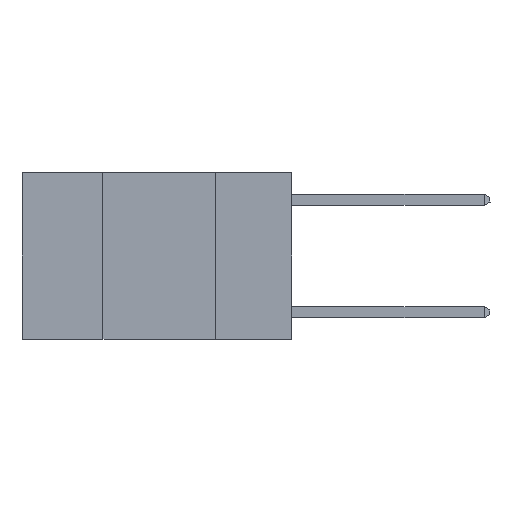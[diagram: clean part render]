
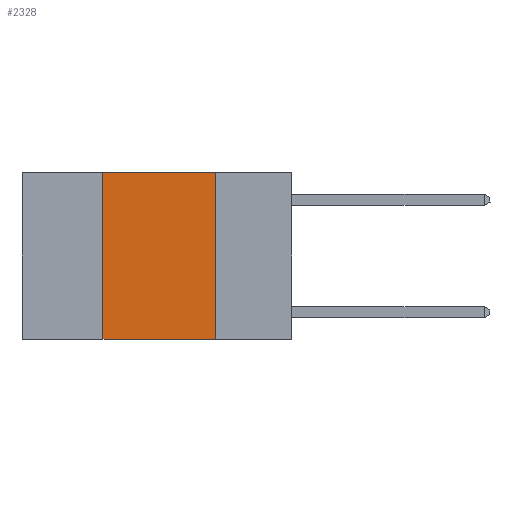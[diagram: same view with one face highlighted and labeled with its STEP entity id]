
A CAD part, left-side view. The second image highlights one B-rep face of the part: STEP entity #2328.
In plain terms, the highlighted planar face has unit normal (-1, 0, 0).
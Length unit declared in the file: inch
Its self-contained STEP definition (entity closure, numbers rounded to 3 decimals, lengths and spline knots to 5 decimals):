
#122 = ORIENTED_EDGE ( 'NONE', *, *, #6256, .F. ) ;
#449 = CARTESIAN_POINT ( 'NONE',  ( 0., 0.42, -0.37 ) ) ;
#525 = LINE ( 'NONE', #4848, #6279 ) ;
#731 = VECTOR ( 'NONE', #2722, 39.37008 ) ;
#1055 = DIRECTION ( 'NONE',  ( 0., -1., 0. ) ) ;
#1073 = CARTESIAN_POINT ( 'NONE',  ( 0., 0.6, -0.37 ) ) ;
#1463 = DIRECTION ( 'NONE',  ( 0., 0., -1. ) ) ;
#1555 = VERTEX_POINT ( 'NONE', #2569 ) ;
#1876 = CARTESIAN_POINT ( 'NONE',  ( 0., 0.42, 0. ) ) ;
#1993 = CARTESIAN_POINT ( 'NONE',  ( 0., 0.6, 0. ) ) ;
#2189 = VERTEX_POINT ( 'NONE', #449 ) ;
#2293 = ORIENTED_EDGE ( 'NONE', *, *, #6608, .F. ) ;
#2328 = ADVANCED_FACE ( 'NONE', ( #3633 ), #8677, .F. ) ;
#2569 = CARTESIAN_POINT ( 'NONE',  ( 0., 0.42, 0. ) ) ;
#2722 = DIRECTION ( 'NONE',  ( 0., 0., 1. ) ) ;
#3633 = FACE_OUTER_BOUND ( 'NONE', #6248, .T. ) ;
#3736 = EDGE_CURVE ( 'NONE', #2189, #7300, #4360, .T. ) ;
#3744 = CARTESIAN_POINT ( 'NONE',  ( 0., 0.17, -0.37 ) ) ;
#4016 = DIRECTION ( 'NONE',  ( 1., 0., 0. ) ) ;
#4308 = VECTOR ( 'NONE', #1463, 39.37008 ) ;
#4360 = LINE ( 'NONE', #1073, #4373 ) ;
#4373 = VECTOR ( 'NONE', #1055, 39.37008 ) ;
#4524 = LINE ( 'NONE', #5296, #4308 ) ;
#4741 = CARTESIAN_POINT ( 'NONE',  ( 0., 0.17, 0. ) ) ;
#4842 = AXIS2_PLACEMENT_3D ( 'NONE', #1993, #4016, #6798 ) ;
#4848 = CARTESIAN_POINT ( 'NONE',  ( 0., 0.6, 0. ) ) ;
#5287 = EDGE_CURVE ( 'NONE', #1555, #5928, #525, .T. ) ;
#5296 = CARTESIAN_POINT ( 'NONE',  ( 0., 0.17, 0. ) ) ;
#5549 = DIRECTION ( 'NONE',  ( 0., -1., 0. ) ) ;
#5928 = VERTEX_POINT ( 'NONE', #4741 ) ;
#6248 = EDGE_LOOP ( 'NONE', ( #2293, #7507, #122, #7807 ) ) ;
#6256 = EDGE_CURVE ( 'NONE', #2189, #1555, #6718, .T. ) ;
#6279 = VECTOR ( 'NONE', #5549, 39.37008 ) ;
#6608 = EDGE_CURVE ( 'NONE', #5928, #7300, #4524, .T. ) ;
#6718 = LINE ( 'NONE', #1876, #731 ) ;
#6798 = DIRECTION ( 'NONE',  ( 0., 0., -1. ) ) ;
#7300 = VERTEX_POINT ( 'NONE', #3744 ) ;
#7507 = ORIENTED_EDGE ( 'NONE', *, *, #5287, .F. ) ;
#7807 = ORIENTED_EDGE ( 'NONE', *, *, #3736, .T. ) ;
#8677 = PLANE ( 'NONE',  #4842 ) ;
